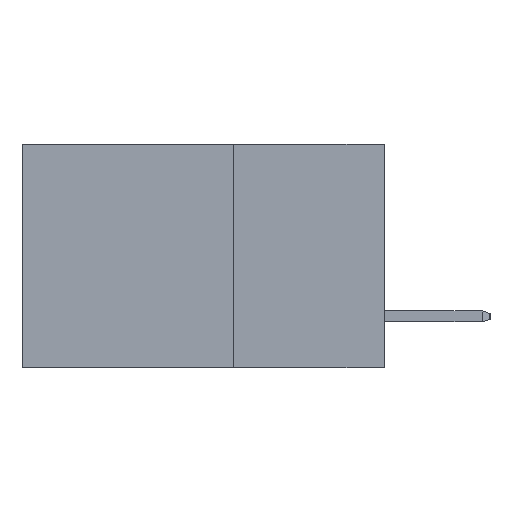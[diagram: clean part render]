
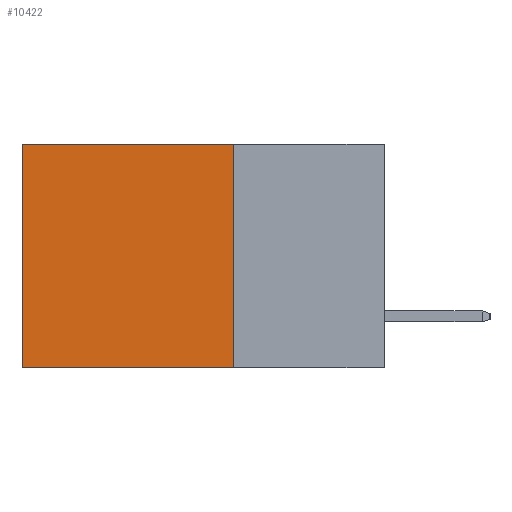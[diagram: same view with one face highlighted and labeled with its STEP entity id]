
A CAD part, left-side view. The second image highlights one B-rep face of the part: STEP entity #10422.
In plain terms, the highlighted planar face has unit normal (-1, 0, 0).
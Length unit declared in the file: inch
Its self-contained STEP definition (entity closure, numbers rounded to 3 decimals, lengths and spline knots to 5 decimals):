
#38 = LINE ( 'NONE', #1105, #15204 ) ;
#329 = CARTESIAN_POINT ( 'NONE',  ( 0.298, 0.6, 0. ) ) ;
#476 = VERTEX_POINT ( 'NONE', #5304 ) ;
#506 = EDGE_CURVE ( 'NONE', #10738, #13698, #7722, .T. ) ;
#1105 = CARTESIAN_POINT ( 'NONE',  ( 0.298, 0.25, 0. ) ) ;
#1354 = LINE ( 'NONE', #12598, #5118 ) ;
#1689 = PLANE ( 'NONE',  #12466 ) ;
#2281 = CARTESIAN_POINT ( 'NONE',  ( 0.298, 0.25, -0.37 ) ) ;
#2284 = ORIENTED_EDGE ( 'NONE', *, *, #11518, .F. ) ;
#3108 = CARTESIAN_POINT ( 'NONE',  ( 0.298, 0.25, 0. ) ) ;
#3531 = CARTESIAN_POINT ( 'NONE',  ( 0.298, 0.25, 0. ) ) ;
#4523 = DIRECTION ( 'NONE',  ( 1., 0., 0. ) ) ;
#5001 = EDGE_LOOP ( 'NONE', ( #14215, #16680, #2284, #15367 ) ) ;
#5015 = FACE_OUTER_BOUND ( 'NONE', #5001, .T. ) ;
#5118 = VECTOR ( 'NONE', #18204, 39.37008 ) ;
#5304 = CARTESIAN_POINT ( 'NONE',  ( 0.298, 0.6, 0. ) ) ;
#5446 = CARTESIAN_POINT ( 'NONE',  ( 0.298, 0.25, -0.37 ) ) ;
#7722 = LINE ( 'NONE', #5446, #14843 ) ;
#7845 = EDGE_CURVE ( 'NONE', #13267, #476, #1354, .T. ) ;
#8404 = LINE ( 'NONE', #329, #12158 ) ;
#8683 = EDGE_CURVE ( 'NONE', #476, #13698, #8404, .T. ) ;
#9584 = DIRECTION ( 'NONE',  ( 0., 0., -1. ) ) ;
#9832 = DIRECTION ( 'NONE',  ( 0., 1., 0. ) ) ;
#10277 = DIRECTION ( 'NONE',  ( 0., 0., -1. ) ) ;
#10422 = ADVANCED_FACE ( 'NONE', ( #5015 ), #1689, .F. ) ;
#10738 = VERTEX_POINT ( 'NONE', #2281 ) ;
#11088 = CARTESIAN_POINT ( 'NONE',  ( 0.298, 0.6, -0.37 ) ) ;
#11518 = EDGE_CURVE ( 'NONE', #13267, #10738, #38, .T. ) ;
#12158 = VECTOR ( 'NONE', #10277, 39.37008 ) ;
#12466 = AXIS2_PLACEMENT_3D ( 'NONE', #3108, #4523, #14453 ) ;
#12598 = CARTESIAN_POINT ( 'NONE',  ( 0.298, 0.25, 0. ) ) ;
#13267 = VERTEX_POINT ( 'NONE', #3531 ) ;
#13698 = VERTEX_POINT ( 'NONE', #11088 ) ;
#14215 = ORIENTED_EDGE ( 'NONE', *, *, #8683, .T. ) ;
#14453 = DIRECTION ( 'NONE',  ( 0., 0., -1. ) ) ;
#14843 = VECTOR ( 'NONE', #9832, 39.37008 ) ;
#15204 = VECTOR ( 'NONE', #9584, 39.37008 ) ;
#15367 = ORIENTED_EDGE ( 'NONE', *, *, #7845, .T. ) ;
#16680 = ORIENTED_EDGE ( 'NONE', *, *, #506, .F. ) ;
#18204 = DIRECTION ( 'NONE',  ( 0., 1., 0. ) ) ;
